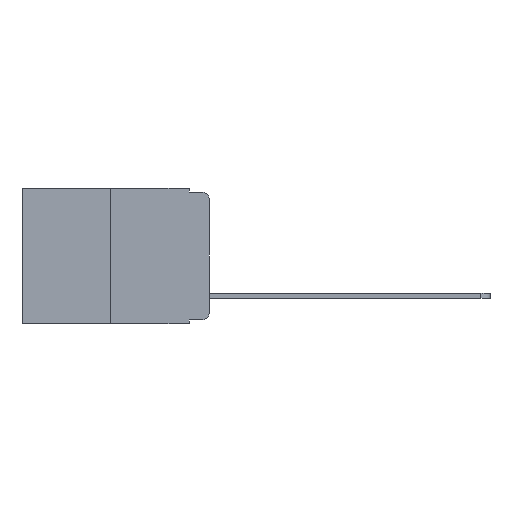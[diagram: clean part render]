
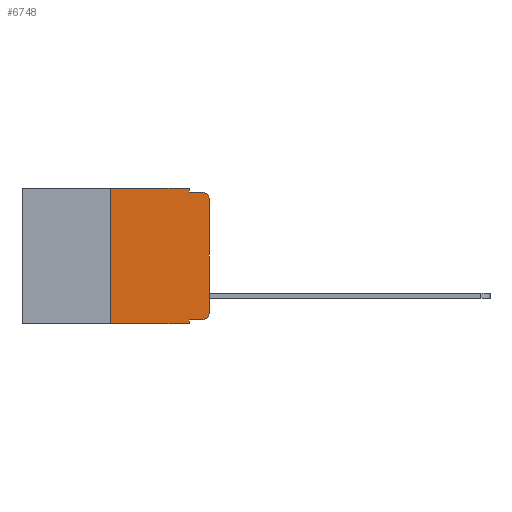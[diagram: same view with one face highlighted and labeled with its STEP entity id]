
A CAD part, left-side view. The second image highlights one B-rep face of the part: STEP entity #6748.
In plain terms, the highlighted planar face has unit normal (-1, 0, 0).
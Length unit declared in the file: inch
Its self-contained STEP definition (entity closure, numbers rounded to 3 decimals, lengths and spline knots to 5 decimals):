
#166 = LINE ( 'NONE', #4440, #2482 ) ;
#272 = ORIENTED_EDGE ( 'NONE', *, *, #4981, .T. ) ;
#511 = LINE ( 'NONE', #4368, #4712 ) ;
#601 = CARTESIAN_POINT ( 'NONE',  ( 0., 0.25, 0. ) ) ;
#696 = CARTESIAN_POINT ( 'NONE',  ( 0., 0., -0.313 ) ) ;
#738 = DIRECTION ( 'NONE',  ( 0., 0., -1. ) ) ;
#860 = AXIS2_PLACEMENT_3D ( 'NONE', #9026, #6871, #2095 ) ;
#1064 = VECTOR ( 'NONE', #2553, 39.37008 ) ;
#1456 = VECTOR ( 'NONE', #5844, 39.37008 ) ;
#1624 = VECTOR ( 'NONE', #2658, 39.37008 ) ;
#1640 = VERTEX_POINT ( 'NONE', #601 ) ;
#1670 = VECTOR ( 'NONE', #8101, 39.37008 ) ;
#2014 = EDGE_CURVE ( 'NONE', #6865, #5666, #5862, .T. ) ;
#2095 = DIRECTION ( 'NONE',  ( 0., 0., -1. ) ) ;
#2151 = CARTESIAN_POINT ( 'NONE',  ( 0., 0., 0. ) ) ;
#2222 = CARTESIAN_POINT ( 'NONE',  ( 0., 0.051, -0.343 ) ) ;
#2482 = VECTOR ( 'NONE', #8947, 39.37008 ) ;
#2553 = DIRECTION ( 'NONE',  ( 0., -1., 0. ) ) ;
#2658 = DIRECTION ( 'NONE',  ( 0., 0., 1. ) ) ;
#2663 = CARTESIAN_POINT ( 'NONE',  ( 0., 0.051, 0. ) ) ;
#2903 = CIRCLE ( 'NONE', #6508, 0.02 ) ;
#2920 = CARTESIAN_POINT ( 'NONE',  ( 0., 0.02, -0.313 ) ) ;
#2946 = ORIENTED_EDGE ( 'NONE', *, *, #6524, .F. ) ;
#2968 = CARTESIAN_POINT ( 'NONE',  ( 0., 0.02, -0.01 ) ) ;
#2989 = VERTEX_POINT ( 'NONE', #2222 ) ;
#3044 = CARTESIAN_POINT ( 'NONE',  ( 0., 0., -0.03 ) ) ;
#3264 = VERTEX_POINT ( 'NONE', #8258 ) ;
#3619 = VERTEX_POINT ( 'NONE', #4667 ) ;
#3637 = ORIENTED_EDGE ( 'NONE', *, *, #2014, .T. ) ;
#3672 = EDGE_CURVE ( 'NONE', #4677, #6865, #3819, .T. ) ;
#3730 = DIRECTION ( 'NONE',  ( 0., 0., -1. ) ) ;
#3819 = LINE ( 'NONE', #2151, #1624 ) ;
#3923 = VERTEX_POINT ( 'NONE', #4366 ) ;
#4098 = EDGE_CURVE ( 'NONE', #3923, #2989, #4334, .T. ) ;
#4151 = ORIENTED_EDGE ( 'NONE', *, *, #8012, .F. ) ;
#4236 = CARTESIAN_POINT ( 'NONE',  ( 0., 0.051, -0.01 ) ) ;
#4334 = LINE ( 'NONE', #7024, #6190 ) ;
#4366 = CARTESIAN_POINT ( 'NONE',  ( 0., 0.25, -0.343 ) ) ;
#4368 = CARTESIAN_POINT ( 'NONE',  ( 0., 0.051, 0. ) ) ;
#4371 = AXIS2_PLACEMENT_3D ( 'NONE', #6727, #7023, #738 ) ;
#4385 = ORIENTED_EDGE ( 'NONE', *, *, #3672, .T. ) ;
#4440 = CARTESIAN_POINT ( 'NONE',  ( 0., 0.051, -0.333 ) ) ;
#4667 = CARTESIAN_POINT ( 'NONE',  ( 0., 0.051, 0. ) ) ;
#4677 = VERTEX_POINT ( 'NONE', #696 ) ;
#4712 = VECTOR ( 'NONE', #5174, 39.37008 ) ;
#4797 = ORIENTED_EDGE ( 'NONE', *, *, #8972, .F. ) ;
#4920 = ORIENTED_EDGE ( 'NONE', *, *, #9439, .F. ) ;
#4981 = EDGE_CURVE ( 'NONE', #3264, #4677, #2903, .T. ) ;
#5113 = DIRECTION ( 'NONE',  ( 0., -1., 0. ) ) ;
#5174 = DIRECTION ( 'NONE',  ( 0., 0., -1. ) ) ;
#5498 = DIRECTION ( 'NONE',  ( 0., 0., 1. ) ) ;
#5666 = VERTEX_POINT ( 'NONE', #2968 ) ;
#5789 = EDGE_LOOP ( 'NONE', ( #4385, #3637, #4920, #4797, #7988, #4151, #8442, #2946, #8071, #272 ) ) ;
#5844 = DIRECTION ( 'NONE',  ( 0., -1., 0. ) ) ;
#5862 = CIRCLE ( 'NONE', #4371, 0.02 ) ;
#6024 = EDGE_CURVE ( 'NONE', #8736, #3264, #166, .T. ) ;
#6190 = VECTOR ( 'NONE', #5113, 39.37008 ) ;
#6508 = AXIS2_PLACEMENT_3D ( 'NONE', #2920, #8347, #3730 ) ;
#6524 = EDGE_CURVE ( 'NONE', #8736, #2989, #9834, .T. ) ;
#6727 = CARTESIAN_POINT ( 'NONE',  ( 0., 0.02, -0.03 ) ) ;
#6748 = ADVANCED_FACE ( 'NONE', ( #9731 ), #9723, .F. ) ;
#6865 = VERTEX_POINT ( 'NONE', #3044 ) ;
#6871 = DIRECTION ( 'NONE',  ( 1., 0., 0. ) ) ;
#6897 = VECTOR ( 'NONE', #5498, 39.37008 ) ;
#7023 = DIRECTION ( 'NONE',  ( -1., 0., 0. ) ) ;
#7024 = CARTESIAN_POINT ( 'NONE',  ( 0., 0.473, -0.343 ) ) ;
#7405 = VERTEX_POINT ( 'NONE', #9054 ) ;
#7449 = LINE ( 'NONE', #10115, #1064 ) ;
#7777 = LINE ( 'NONE', #4236, #1456 ) ;
#7988 = ORIENTED_EDGE ( 'NONE', *, *, #8859, .F. ) ;
#8012 = EDGE_CURVE ( 'NONE', #3923, #1640, #8830, .T. ) ;
#8071 = ORIENTED_EDGE ( 'NONE', *, *, #6024, .T. ) ;
#8101 = DIRECTION ( 'NONE',  ( 0., 0., -1. ) ) ;
#8258 = CARTESIAN_POINT ( 'NONE',  ( 0., 0.02, -0.333 ) ) ;
#8347 = DIRECTION ( 'NONE',  ( -1., 0., 0. ) ) ;
#8442 = ORIENTED_EDGE ( 'NONE', *, *, #4098, .T. ) ;
#8736 = VERTEX_POINT ( 'NONE', #9315 ) ;
#8830 = LINE ( 'NONE', #9855, #6897 ) ;
#8859 = EDGE_CURVE ( 'NONE', #1640, #3619, #7449, .T. ) ;
#8947 = DIRECTION ( 'NONE',  ( 0., -1., 0. ) ) ;
#8972 = EDGE_CURVE ( 'NONE', #3619, #7405, #511, .T. ) ;
#9026 = CARTESIAN_POINT ( 'NONE',  ( 0., 0.473, 0. ) ) ;
#9054 = CARTESIAN_POINT ( 'NONE',  ( 0., 0.051, -0.01 ) ) ;
#9315 = CARTESIAN_POINT ( 'NONE',  ( 0., 0.051, -0.333 ) ) ;
#9439 = EDGE_CURVE ( 'NONE', #7405, #5666, #7777, .T. ) ;
#9723 = PLANE ( 'NONE',  #860 ) ;
#9731 = FACE_OUTER_BOUND ( 'NONE', #5789, .T. ) ;
#9834 = LINE ( 'NONE', #2663, #1670 ) ;
#9855 = CARTESIAN_POINT ( 'NONE',  ( 0., 0.25, 0. ) ) ;
#10115 = CARTESIAN_POINT ( 'NONE',  ( 0., 0.473, 0. ) ) ;
